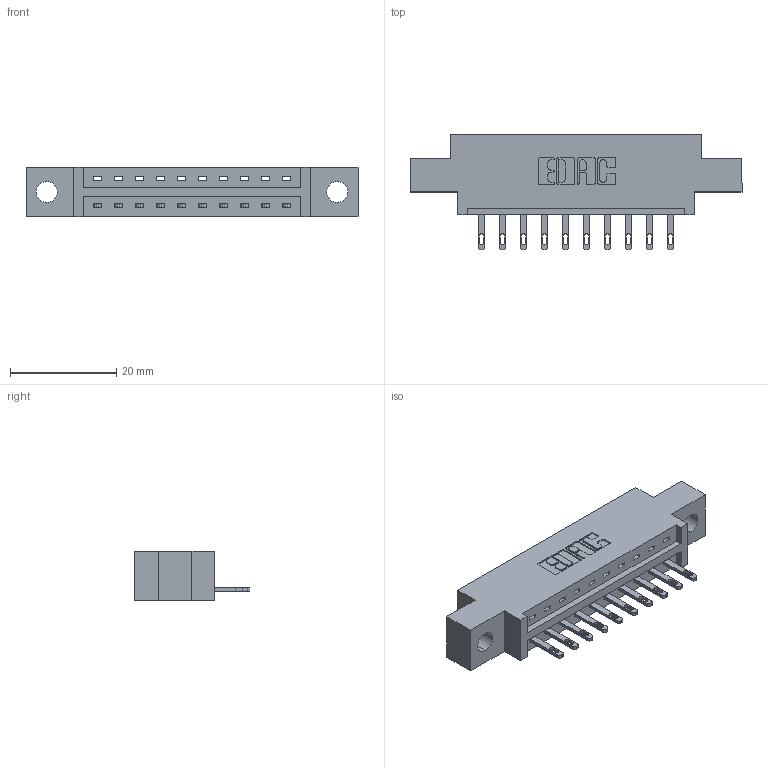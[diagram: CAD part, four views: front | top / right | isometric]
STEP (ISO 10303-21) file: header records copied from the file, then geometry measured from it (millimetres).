
FILE_DESCRIPTION (( 'STEP AP203' ), '1' );
FILE_NAME ('887-010-500-604.STEP', '2020-09-20T16:04:59', ( '' ), ( '' ), 'SwSTEP 2.0', 'SolidWorks 2020', '' );
FILE_SCHEMA (( 'CONFIG_CONTROL_DESIGN' ));
Length unit declared in the file: inch
Products named in the file (3): 345-292-001_345-293-100; 837 Part_0.170 Offset - 0.156 Dia-TH; 887-010-500-604
Assembly tree (11 placements, depth 2):
  887-010-500-604
    837 Part_0.170 Offset - 0.156 Dia-TH
    345-292-001_345-293-100  x10
Bounding box: 62.64 x 21.85 x 9.4 mm (x, y, z)
Volume: 5910.4 mm3; surface area: 5845 mm2
Topology: 11 solids, 11 shells, 698 faces, 2123 edges, 1414 vertices
Faces by surface type: plane 474, cylinder 224
Entity records: 11637 total; most frequent: CARTESIAN_POINT 2032, ORIENTED_EDGE 1978, DIRECTION 1777, EDGE_CURVE 989, LINE 857, VECTOR 857, VERTEX_POINT 658, AXIS2_PLACEMENT_3D 460
